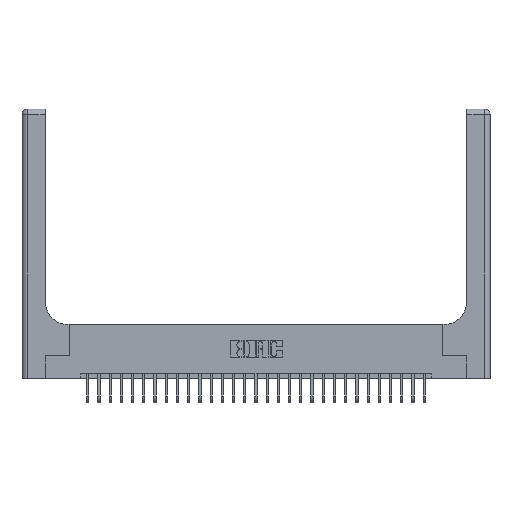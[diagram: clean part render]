
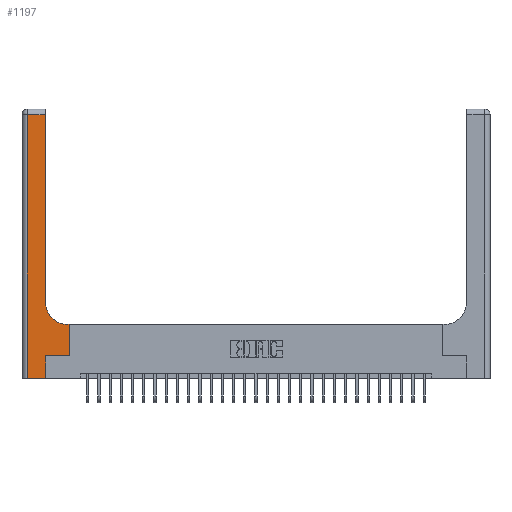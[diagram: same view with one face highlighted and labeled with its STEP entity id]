
A CAD part, top view. The second image highlights one B-rep face of the part: STEP entity #1197.
In plain terms, the highlighted planar face has unit normal (0, 0, 1).
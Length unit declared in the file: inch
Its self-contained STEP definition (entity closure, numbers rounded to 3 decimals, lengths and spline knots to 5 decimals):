
#434 = VECTOR ( 'NONE', #16908, 39.37008 ) ;
#1197 = ADVANCED_FACE ( 'NONE', ( #22612 ), #4299, .F. ) ;
#1837 = LINE ( 'NONE', #6119, #9391 ) ;
#2343 = CARTESIAN_POINT ( 'NONE',  ( 0.265, 0., 0.37 ) ) ;
#2358 = CARTESIAN_POINT ( 'NONE',  ( 0.06, 3., 0.37 ) ) ;
#2473 = CARTESIAN_POINT ( 'NONE',  ( 0.265, 0., 0.37 ) ) ;
#2514 = EDGE_CURVE ( 'NONE', #7541, #3823, #4909, .T. ) ;
#3333 = ORIENTED_EDGE ( 'NONE', *, *, #2514, .T. ) ;
#3823 = VERTEX_POINT ( 'NONE', #11659 ) ;
#4213 = VECTOR ( 'NONE', #10446, 39.37008 ) ;
#4299 = PLANE ( 'NONE',  #17023 ) ;
#4339 = CARTESIAN_POINT ( 'NONE',  ( 0.06, 0., 0.37 ) ) ;
#4382 = DIRECTION ( 'NONE',  ( 0., -1., 0. ) ) ;
#4441 = ORIENTED_EDGE ( 'NONE', *, *, #12478, .T. ) ;
#4462 = CARTESIAN_POINT ( 'NONE',  ( 0., 2.94, 0.37 ) ) ;
#4584 = LINE ( 'NONE', #12727, #4213 ) ;
#4909 = LINE ( 'NONE', #25204, #7813 ) ;
#5174 = VECTOR ( 'NONE', #6696, 39.37008 ) ;
#5897 = EDGE_CURVE ( 'NONE', #3823, #12910, #18728, .T. ) ;
#6119 = CARTESIAN_POINT ( 'NONE',  ( 0.265, 0.25, 0.37 ) ) ;
#6419 = DIRECTION ( 'NONE',  ( 0., 0., -1. ) ) ;
#6696 = DIRECTION ( 'NONE',  ( -1., 0., 0. ) ) ;
#6886 = EDGE_CURVE ( 'NONE', #23967, #24328, #25697, .T. ) ;
#6913 = VECTOR ( 'NONE', #7649, 39.37008 ) ;
#7541 = VERTEX_POINT ( 'NONE', #26197 ) ;
#7649 = DIRECTION ( 'NONE',  ( 1., 0., 0. ) ) ;
#7813 = VECTOR ( 'NONE', #8895, 39.37008 ) ;
#7963 = EDGE_CURVE ( 'NONE', #21724, #23967, #1837, .T. ) ;
#8420 = VERTEX_POINT ( 'NONE', #2343 ) ;
#8566 = ORIENTED_EDGE ( 'NONE', *, *, #5897, .T. ) ;
#8872 = ORIENTED_EDGE ( 'NONE', *, *, #14251, .T. ) ;
#8895 = DIRECTION ( 'NONE',  ( 0., 1., 0. ) ) ;
#8950 = DIRECTION ( 'NONE',  ( 0., 0., -1. ) ) ;
#9391 = VECTOR ( 'NONE', #26161, 39.37008 ) ;
#9629 = CIRCLE ( 'NONE', #23317, 0.25 ) ;
#10446 = DIRECTION ( 'NONE',  ( -1., 0., 0. ) ) ;
#11015 = LINE ( 'NONE', #2473, #434 ) ;
#11351 = DIRECTION ( 'NONE',  ( 1., 0., 0. ) ) ;
#11480 = CARTESIAN_POINT ( 'NONE',  ( 0.51, 0.85, 0.37 ) ) ;
#11659 = CARTESIAN_POINT ( 'NONE',  ( 0.26, 2.94, 0.37 ) ) ;
#11662 = DIRECTION ( 'NONE',  ( 0., 1., 0. ) ) ;
#11848 = ORIENTED_EDGE ( 'NONE', *, *, #26157, .T. ) ;
#12038 = CARTESIAN_POINT ( 'NONE',  ( 0., 3., 0.37 ) ) ;
#12116 = VECTOR ( 'NONE', #4382, 39.37008 ) ;
#12234 = LINE ( 'NONE', #2358, #12116 ) ;
#12478 = EDGE_CURVE ( 'NONE', #18613, #8420, #25690, .T. ) ;
#12727 = CARTESIAN_POINT ( 'NONE',  ( 0.26, 0.6, 0.37 ) ) ;
#12836 = ORIENTED_EDGE ( 'NONE', *, *, #7963, .T. ) ;
#12910 = VERTEX_POINT ( 'NONE', #19891 ) ;
#13984 = CARTESIAN_POINT ( 'NONE',  ( 0.528, 0.25, 0.37 ) ) ;
#14251 = EDGE_CURVE ( 'NONE', #24328, #25861, #4584, .T. ) ;
#14576 = DIRECTION ( 'NONE',  ( -1., 0., 0. ) ) ;
#16908 = DIRECTION ( 'NONE',  ( 0., 1., 0. ) ) ;
#17023 = AXIS2_PLACEMENT_3D ( 'NONE', #12038, #6419, #14576 ) ;
#17264 = CARTESIAN_POINT ( 'NONE',  ( 0.51, 0.6, 0.37 ) ) ;
#17698 = CARTESIAN_POINT ( 'NONE',  ( 0.528, 0.6, 0.37 ) ) ;
#18154 = EDGE_CURVE ( 'NONE', #8420, #21724, #11015, .T. ) ;
#18613 = VERTEX_POINT ( 'NONE', #4339 ) ;
#18728 = LINE ( 'NONE', #4462, #5174 ) ;
#19329 = EDGE_LOOP ( 'NONE', ( #3333, #8566, #22091, #4441, #25413, #12836, #25797, #8872, #11848 ) ) ;
#19891 = CARTESIAN_POINT ( 'NONE',  ( 0.06, 2.94, 0.37 ) ) ;
#21724 = VERTEX_POINT ( 'NONE', #21823 ) ;
#21823 = CARTESIAN_POINT ( 'NONE',  ( 0.265, 0.25, 0.37 ) ) ;
#22091 = ORIENTED_EDGE ( 'NONE', *, *, #24101, .T. ) ;
#22612 = FACE_OUTER_BOUND ( 'NONE', #19329, .T. ) ;
#23317 = AXIS2_PLACEMENT_3D ( 'NONE', #11480, #8950, #11351 ) ;
#23967 = VERTEX_POINT ( 'NONE', #13984 ) ;
#24101 = EDGE_CURVE ( 'NONE', #12910, #18613, #12234, .T. ) ;
#24328 = VERTEX_POINT ( 'NONE', #17698 ) ;
#24336 = VECTOR ( 'NONE', #11662, 39.37008 ) ;
#25204 = CARTESIAN_POINT ( 'NONE',  ( 0.26, 3., 0.37 ) ) ;
#25413 = ORIENTED_EDGE ( 'NONE', *, *, #18154, .T. ) ;
#25690 = LINE ( 'NONE', #25935, #6913 ) ;
#25697 = LINE ( 'NONE', #25940, #24336 ) ;
#25797 = ORIENTED_EDGE ( 'NONE', *, *, #6886, .T. ) ;
#25861 = VERTEX_POINT ( 'NONE', #17264 ) ;
#25935 = CARTESIAN_POINT ( 'NONE',  ( 0., 0., 0.37 ) ) ;
#25940 = CARTESIAN_POINT ( 'NONE',  ( 0.528, 0.25, 0.37 ) ) ;
#26157 = EDGE_CURVE ( 'NONE', #25861, #7541, #9629, .T. ) ;
#26161 = DIRECTION ( 'NONE',  ( 1., 0., 0. ) ) ;
#26197 = CARTESIAN_POINT ( 'NONE',  ( 0.26, 0.85, 0.37 ) ) ;
